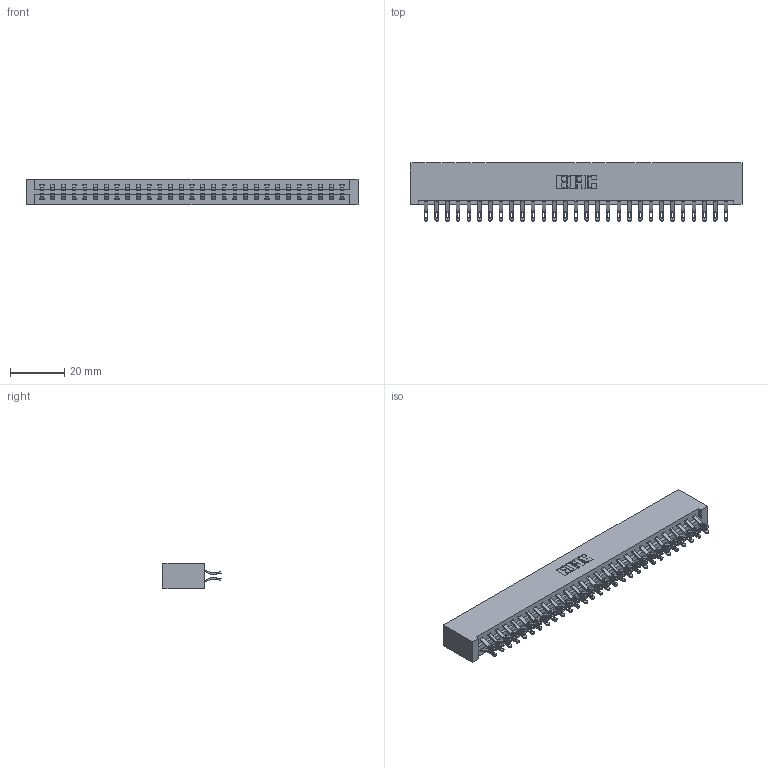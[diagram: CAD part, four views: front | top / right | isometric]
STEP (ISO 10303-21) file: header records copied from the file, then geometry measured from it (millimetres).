
FILE_DESCRIPTION (( 'STEP AP203' ), '1' );
FILE_NAME ('387-058-555-201.STEP', '2018-09-21T01:53:58', ( '' ), ( '' ), 'SwSTEP 2.0', 'SolidWorks 2016', '' );
FILE_SCHEMA (( 'CONFIG_CONTROL_DESIGN' ));
Length unit declared in the file: inch
Products named in the file (3): 337 Part_No Mounting Lugs; 345-292-001_555 Tail; 387-058-555-201
Assembly tree (59 placements, depth 2):
  387-058-555-201
    337 Part_No Mounting Lugs
    345-292-001_555 Tail  x58
Bounding box: 122.78 x 21.47 x 9.4 mm (x, y, z)
Volume: 13695.8 mm3; surface area: 16047 mm2
Topology: 59 solids, 59 shells, 3586 faces, 11249 edges, 7498 vertices
Faces by surface type: plane 2154, cylinder 1432
Entity records: 24215 total; most frequent: CARTESIAN_POINT 4124, ORIENTED_EDGE 4030, DIRECTION 3495, EDGE_CURVE 2015, VECTOR 1875, LINE 1875, VERTEX_POINT 1342, AXIS2_PLACEMENT_3D 810
